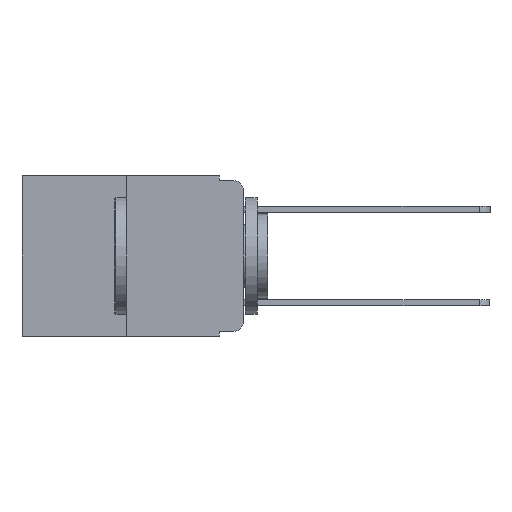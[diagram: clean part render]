
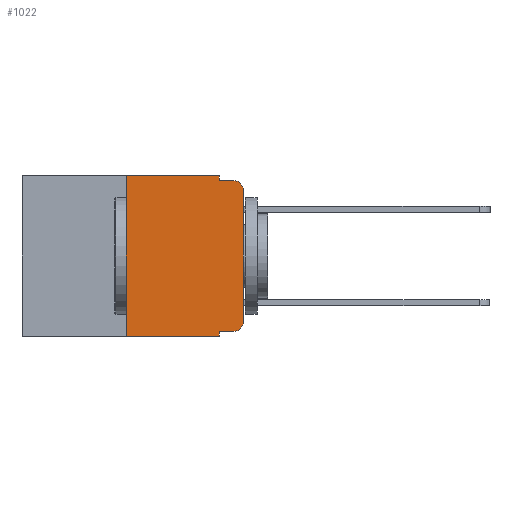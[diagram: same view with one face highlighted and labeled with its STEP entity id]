
A CAD part, left-side view. The second image highlights one B-rep face of the part: STEP entity #1022.
In plain terms, the highlighted planar face has unit normal (-1, 0, 0).
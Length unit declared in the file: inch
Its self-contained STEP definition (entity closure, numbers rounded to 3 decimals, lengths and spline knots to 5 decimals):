
#188 = DIRECTION ( 'NONE',  ( 0., 0., 1. ) ) ;
#237 = AXIS2_PLACEMENT_3D ( 'NONE', #1756, #3305, #3018 ) ;
#242 = DIRECTION ( 'NONE',  ( 0., -1., 0. ) ) ;
#295 = DIRECTION ( 'NONE',  ( 0., 0., -1. ) ) ;
#622 = VECTOR ( 'NONE', #1838, 39.37008 ) ;
#1022 = ADVANCED_FACE ( 'NONE', ( #6558 ), #1431, .F. ) ;
#1128 = DIRECTION ( 'NONE',  ( 0., 0., -1. ) ) ;
#1326 = VERTEX_POINT ( 'NONE', #6526 ) ;
#1431 = PLANE ( 'NONE',  #237 ) ;
#1556 = VECTOR ( 'NONE', #1128, 39.37008 ) ;
#1756 = CARTESIAN_POINT ( 'NONE',  ( 0., 0.473, 0. ) ) ;
#1838 = DIRECTION ( 'NONE',  ( 0., -1., 0. ) ) ;
#1888 = VECTOR ( 'NONE', #6411, 39.37008 ) ;
#2241 = CARTESIAN_POINT ( 'NONE',  ( 0., 0.25, 0. ) ) ;
#2442 = ORIENTED_EDGE ( 'NONE', *, *, #6287, .F. ) ;
#2656 = VERTEX_POINT ( 'NONE', #8567 ) ;
#3018 = DIRECTION ( 'NONE',  ( 0., 0., -1. ) ) ;
#3027 = ORIENTED_EDGE ( 'NONE', *, *, #6288, .T. ) ;
#3092 = AXIS2_PLACEMENT_3D ( 'NONE', #3356, #9874, #4381 ) ;
#3112 = LINE ( 'NONE', #3567, #5504 ) ;
#3286 = CARTESIAN_POINT ( 'NONE',  ( 0., 0.051, -0.01 ) ) ;
#3305 = DIRECTION ( 'NONE',  ( 1., 0., 0. ) ) ;
#3330 = ORIENTED_EDGE ( 'NONE', *, *, #6254, .T. ) ;
#3356 = CARTESIAN_POINT ( 'NONE',  ( 0., 0.02, -0.313 ) ) ;
#3400 = CARTESIAN_POINT ( 'NONE',  ( 0., 0.051, -0.01 ) ) ;
#3455 = VERTEX_POINT ( 'NONE', #6777 ) ;
#3518 = ORIENTED_EDGE ( 'NONE', *, *, #6308, .T. ) ;
#3567 = CARTESIAN_POINT ( 'NONE',  ( 0., 0.473, 0. ) ) ;
#3751 = LINE ( 'NONE', #10382, #622 ) ;
#4381 = DIRECTION ( 'NONE',  ( 0., 0., -1. ) ) ;
#4516 = CARTESIAN_POINT ( 'NONE',  ( 0., 0., 0. ) ) ;
#4751 = VERTEX_POINT ( 'NONE', #9014 ) ;
#4960 = EDGE_LOOP ( 'NONE', ( #3518, #3027, #2442, #5385, #8819, #8504, #8176, #9447, #3330, #5952 ) ) ;
#5025 = LINE ( 'NONE', #2241, #9344 ) ;
#5139 = AXIS2_PLACEMENT_3D ( 'NONE', #11495, #6497, #295 ) ;
#5385 = ORIENTED_EDGE ( 'NONE', *, *, #6269, .F. ) ;
#5402 = CARTESIAN_POINT ( 'NONE',  ( 0., 0.051, 0. ) ) ;
#5504 = VECTOR ( 'NONE', #9249, 39.37008 ) ;
#5952 = ORIENTED_EDGE ( 'NONE', *, *, #6250, .T. ) ;
#6054 = EDGE_CURVE ( 'NONE', #3455, #10592, #3751, .T. ) ;
#6250 = EDGE_CURVE ( 'NONE', #2656, #9998, #9850, .T. ) ;
#6254 = EDGE_CURVE ( 'NONE', #11874, #2656, #11651, .T. ) ;
#6256 = EDGE_CURVE ( 'NONE', #11874, #10592, #9593, .T. ) ;
#6266 = EDGE_CURVE ( 'NONE', #3455, #1326, #5025, .T. ) ;
#6269 = EDGE_CURVE ( 'NONE', #11928, #7227, #7070, .T. ) ;
#6287 = EDGE_CURVE ( 'NONE', #7227, #10170, #11189, .T. ) ;
#6288 = EDGE_CURVE ( 'NONE', #4751, #10170, #9101, .T. ) ;
#6308 = EDGE_CURVE ( 'NONE', #9998, #4751, #10948, .T. ) ;
#6366 = EDGE_CURVE ( 'NONE', #1326, #11928, #3112, .T. ) ;
#6411 = DIRECTION ( 'NONE',  ( 0., 0., -1. ) ) ;
#6497 = DIRECTION ( 'NONE',  ( -1., 0., 0. ) ) ;
#6526 = CARTESIAN_POINT ( 'NONE',  ( 0., 0.25, 0. ) ) ;
#6558 = FACE_OUTER_BOUND ( 'NONE', #4960, .T. ) ;
#6741 = VECTOR ( 'NONE', #242, 39.37008 ) ;
#6777 = CARTESIAN_POINT ( 'NONE',  ( 0., 0.25, -0.343 ) ) ;
#7070 = LINE ( 'NONE', #11433, #1556 ) ;
#7227 = VERTEX_POINT ( 'NONE', #3286 ) ;
#7372 = VECTOR ( 'NONE', #8255, 39.37008 ) ;
#8176 = ORIENTED_EDGE ( 'NONE', *, *, #6054, .T. ) ;
#8255 = DIRECTION ( 'NONE',  ( 0., -1., 0. ) ) ;
#8504 = ORIENTED_EDGE ( 'NONE', *, *, #6266, .F. ) ;
#8567 = CARTESIAN_POINT ( 'NONE',  ( 0., 0.02, -0.333 ) ) ;
#8819 = ORIENTED_EDGE ( 'NONE', *, *, #6366, .F. ) ;
#8848 = VECTOR ( 'NONE', #9178, 39.37008 ) ;
#9014 = CARTESIAN_POINT ( 'NONE',  ( 0., 0., -0.03 ) ) ;
#9077 = CARTESIAN_POINT ( 'NONE',  ( 0., 0.051, -0.333 ) ) ;
#9101 = CIRCLE ( 'NONE', #5139, 0.02 ) ;
#9178 = DIRECTION ( 'NONE',  ( 0., 0., 1. ) ) ;
#9249 = DIRECTION ( 'NONE',  ( 0., -1., 0. ) ) ;
#9344 = VECTOR ( 'NONE', #188, 39.37008 ) ;
#9447 = ORIENTED_EDGE ( 'NONE', *, *, #6256, .F. ) ;
#9471 = CARTESIAN_POINT ( 'NONE',  ( 0., 0., -0.313 ) ) ;
#9593 = LINE ( 'NONE', #5402, #1888 ) ;
#9850 = CIRCLE ( 'NONE', #3092, 0.02 ) ;
#9874 = DIRECTION ( 'NONE',  ( -1., 0., 0. ) ) ;
#9998 = VERTEX_POINT ( 'NONE', #9471 ) ;
#10170 = VERTEX_POINT ( 'NONE', #11872 ) ;
#10382 = CARTESIAN_POINT ( 'NONE',  ( 0., 0.473, -0.343 ) ) ;
#10592 = VERTEX_POINT ( 'NONE', #12005 ) ;
#10755 = CARTESIAN_POINT ( 'NONE',  ( 0., 0.051, -0.333 ) ) ;
#10948 = LINE ( 'NONE', #4516, #8848 ) ;
#11189 = LINE ( 'NONE', #3400, #6741 ) ;
#11433 = CARTESIAN_POINT ( 'NONE',  ( 0., 0.051, 0. ) ) ;
#11495 = CARTESIAN_POINT ( 'NONE',  ( 0., 0.02, -0.03 ) ) ;
#11509 = CARTESIAN_POINT ( 'NONE',  ( 0., 0.051, 0. ) ) ;
#11651 = LINE ( 'NONE', #9077, #7372 ) ;
#11872 = CARTESIAN_POINT ( 'NONE',  ( 0., 0.02, -0.01 ) ) ;
#11874 = VERTEX_POINT ( 'NONE', #10755 ) ;
#11928 = VERTEX_POINT ( 'NONE', #11509 ) ;
#12005 = CARTESIAN_POINT ( 'NONE',  ( 0., 0.051, -0.343 ) ) ;
